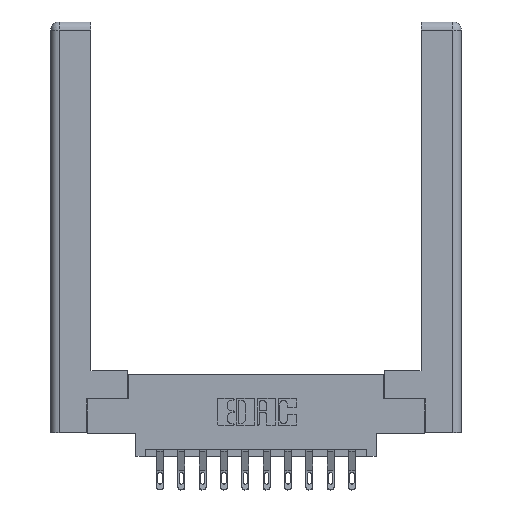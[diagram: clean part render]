
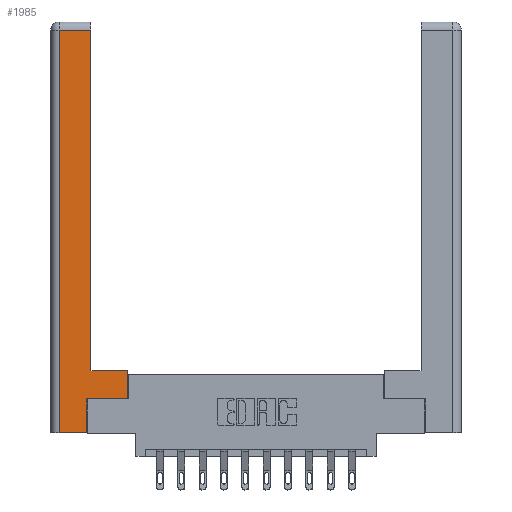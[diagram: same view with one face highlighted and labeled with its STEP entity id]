
A CAD part, top view. The second image highlights one B-rep face of the part: STEP entity #1985.
In plain terms, the highlighted planar face has unit normal (0, 0, 1).
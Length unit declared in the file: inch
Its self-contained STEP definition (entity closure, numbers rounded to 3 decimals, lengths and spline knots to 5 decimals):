
#11 = EDGE_CURVE ( 'NONE', #14127, #9448, #11806, .T. ) ;
#46 = VERTEX_POINT ( 'NONE', #5437 ) ;
#200 = DIRECTION ( 'NONE',  ( -1., 0., 0. ) ) ;
#816 = CARTESIAN_POINT ( 'NONE',  ( 0.565, 0.245, 0. ) ) ;
#990 = ORIENTED_EDGE ( 'NONE', *, *, #10611, .T. ) ;
#1027 = DIRECTION ( 'NONE',  ( -1., 0., 0. ) ) ;
#1055 = ORIENTED_EDGE ( 'NONE', *, *, #10725, .T. ) ;
#1123 = VECTOR ( 'NONE', #2600, 39.37008 ) ;
#1418 = VECTOR ( 'NONE', #9983, 39.37008 ) ;
#1818 = CARTESIAN_POINT ( 'NONE',  ( 0.0615, 0., 0. ) ) ;
#1948 = PLANE ( 'NONE',  #12656 ) ;
#1985 = ADVANCED_FACE ( 'NONE', ( #14448 ), #1948, .F. ) ;
#2166 = CARTESIAN_POINT ( 'NONE',  ( 0.295, 0.45, 0. ) ) ;
#2388 = ORIENTED_EDGE ( 'NONE', *, *, #10447, .T. ) ;
#2451 = ORIENTED_EDGE ( 'NONE', *, *, #9128, .T. ) ;
#2496 = CARTESIAN_POINT ( 'NONE',  ( 0.295, 0.45, 0. ) ) ;
#2557 = VECTOR ( 'NONE', #1027, 39.37008 ) ;
#2600 = DIRECTION ( 'NONE',  ( 0., 1., 0. ) ) ;
#2834 = CARTESIAN_POINT ( 'NONE',  ( 0.295, 2.94, 0. ) ) ;
#2937 = DIRECTION ( 'NONE',  ( 1., 0., 0. ) ) ;
#3438 = VERTEX_POINT ( 'NONE', #1818 ) ;
#3965 = VERTEX_POINT ( 'NONE', #11576 ) ;
#4010 = EDGE_CURVE ( 'NONE', #13316, #3965, #11666, .T. ) ;
#4161 = CARTESIAN_POINT ( 'NONE',  ( 0.295, 3., 0. ) ) ;
#4163 = ORIENTED_EDGE ( 'NONE', *, *, #11, .T. ) ;
#4270 = LINE ( 'NONE', #8887, #4988 ) ;
#4588 = CARTESIAN_POINT ( 'NONE',  ( 0.0615, 2.94, 0. ) ) ;
#4988 = VECTOR ( 'NONE', #8142, 39.37008 ) ;
#5378 = DIRECTION ( 'NONE',  ( 0., 1., 0. ) ) ;
#5437 = CARTESIAN_POINT ( 'NONE',  ( 0.565, 0.45, 0. ) ) ;
#5893 = CARTESIAN_POINT ( 'NONE',  ( 0.565, 0.245, 0. ) ) ;
#6286 = CARTESIAN_POINT ( 'NONE',  ( 0.265, 0., 0. ) ) ;
#6328 = EDGE_CURVE ( 'NONE', #3965, #10413, #14645, .T. ) ;
#6395 = VECTOR ( 'NONE', #200, 39.37008 ) ;
#6554 = CARTESIAN_POINT ( 'NONE',  ( 0., 0., 0. ) ) ;
#8113 = CARTESIAN_POINT ( 'NONE',  ( 0.565, 0.45, 0. ) ) ;
#8142 = DIRECTION ( 'NONE',  ( 0., -1., 0. ) ) ;
#8215 = LINE ( 'NONE', #2496, #6395 ) ;
#8319 = VECTOR ( 'NONE', #12320, 39.37008 ) ;
#8355 = LINE ( 'NONE', #4588, #2557 ) ;
#8566 = LINE ( 'NONE', #9883, #14206 ) ;
#8887 = CARTESIAN_POINT ( 'NONE',  ( 0.0615, 0., 0. ) ) ;
#8952 = DIRECTION ( 'NONE',  ( 0., 0., -1. ) ) ;
#9128 = EDGE_CURVE ( 'NONE', #11986, #3438, #4270, .T. ) ;
#9448 = VERTEX_POINT ( 'NONE', #2834 ) ;
#9655 = ORIENTED_EDGE ( 'NONE', *, *, #11229, .T. ) ;
#9883 = CARTESIAN_POINT ( 'NONE',  ( 0.265, 0., 0. ) ) ;
#9983 = DIRECTION ( 'NONE',  ( 1., 0., 0. ) ) ;
#10413 = VERTEX_POINT ( 'NONE', #5893 ) ;
#10447 = EDGE_CURVE ( 'NONE', #46, #14127, #8215, .T. ) ;
#10611 = EDGE_CURVE ( 'NONE', #3438, #13316, #8566, .T. ) ;
#10725 = EDGE_CURVE ( 'NONE', #10413, #46, #12052, .T. ) ;
#11206 = ORIENTED_EDGE ( 'NONE', *, *, #6328, .T. ) ;
#11229 = EDGE_CURVE ( 'NONE', #9448, #11986, #8355, .T. ) ;
#11416 = CARTESIAN_POINT ( 'NONE',  ( 0.0615, 2.94, 0. ) ) ;
#11576 = CARTESIAN_POINT ( 'NONE',  ( 0.265, 0.245, 0. ) ) ;
#11666 = LINE ( 'NONE', #11871, #1123 ) ;
#11806 = LINE ( 'NONE', #4161, #8319 ) ;
#11859 = ORIENTED_EDGE ( 'NONE', *, *, #4010, .T. ) ;
#11871 = CARTESIAN_POINT ( 'NONE',  ( 0.265, 0.245, 0. ) ) ;
#11986 = VERTEX_POINT ( 'NONE', #11416 ) ;
#12052 = LINE ( 'NONE', #8113, #13867 ) ;
#12320 = DIRECTION ( 'NONE',  ( 0., 1., 0. ) ) ;
#12656 = AXIS2_PLACEMENT_3D ( 'NONE', #6554, #8952, #14749 ) ;
#13316 = VERTEX_POINT ( 'NONE', #6286 ) ;
#13867 = VECTOR ( 'NONE', #5378, 39.37008 ) ;
#14127 = VERTEX_POINT ( 'NONE', #2166 ) ;
#14206 = VECTOR ( 'NONE', #2937, 39.37008 ) ;
#14448 = FACE_OUTER_BOUND ( 'NONE', #14668, .T. ) ;
#14645 = LINE ( 'NONE', #816, #1418 ) ;
#14668 = EDGE_LOOP ( 'NONE', ( #4163, #9655, #2451, #990, #11859, #11206, #1055, #2388 ) ) ;
#14749 = DIRECTION ( 'NONE',  ( -1., 0., 0. ) ) ;
